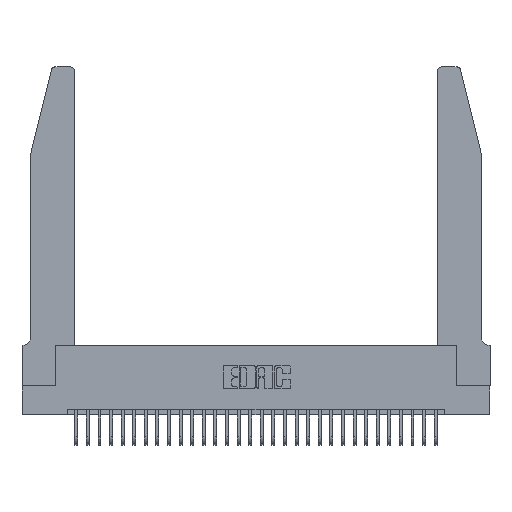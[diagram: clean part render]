
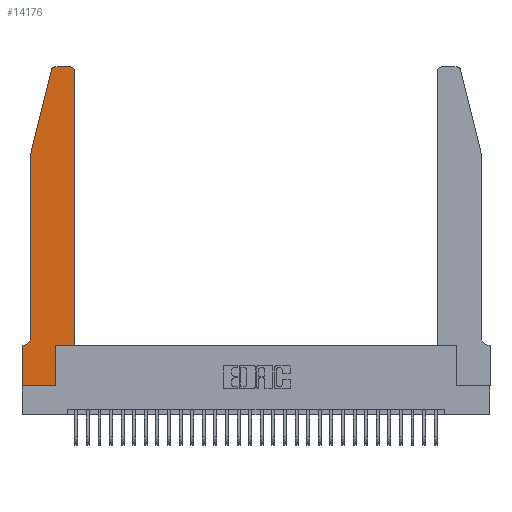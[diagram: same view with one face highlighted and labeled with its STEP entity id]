
A CAD part, top view. The second image highlights one B-rep face of the part: STEP entity #14176.
In plain terms, the highlighted planar face has unit normal (0, 0, 1).
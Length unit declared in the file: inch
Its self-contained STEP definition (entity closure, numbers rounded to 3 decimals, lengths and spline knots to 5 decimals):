
#219 = VERTEX_POINT ( 'NONE', #13088 ) ;
#711 = CARTESIAN_POINT ( 'NONE',  ( 0., 0.35, 0.37 ) ) ;
#771 = CARTESIAN_POINT ( 'NONE',  ( 0.284, 2.72, 0.37 ) ) ;
#917 = AXIS2_PLACEMENT_3D ( 'NONE', #13949, #31653, #6155 ) ;
#1237 = LINE ( 'NONE', #27225, #2818 ) ;
#1404 = EDGE_CURVE ( 'NONE', #24025, #219, #1237, .T. ) ;
#1499 = CARTESIAN_POINT ( 'NONE',  ( 0.0755, 2., 0.37 ) ) ;
#2459 = CARTESIAN_POINT ( 'NONE',  ( 0.25487, 2.72718, 0.37 ) ) ;
#2487 = ORIENTED_EDGE ( 'NONE', *, *, #15381, .T. ) ;
#2818 = VECTOR ( 'NONE', #19490, 39.37008 ) ;
#2945 = ORIENTED_EDGE ( 'NONE', *, *, #10457, .T. ) ;
#2950 = PLANE ( 'NONE',  #24536 ) ;
#3220 = DIRECTION ( 'NONE',  ( -1., 0., 0. ) ) ;
#3922 = EDGE_CURVE ( 'NONE', #29432, #16314, #8284, .T. ) ;
#4212 = DIRECTION ( 'NONE',  ( 0., -1., 0. ) ) ;
#4270 = ORIENTED_EDGE ( 'NONE', *, *, #27706, .T. ) ;
#4544 = CARTESIAN_POINT ( 'NONE',  ( 0., 0., 0.37 ) ) ;
#5168 = VERTEX_POINT ( 'NONE', #10893 ) ;
#5199 = EDGE_CURVE ( 'NONE', #18612, #29432, #10990, .T. ) ;
#5569 = LINE ( 'NONE', #15874, #29776 ) ;
#5787 = CIRCLE ( 'NONE', #917, 0.03 ) ;
#5905 = DIRECTION ( 'NONE',  ( 1., 0., 0. ) ) ;
#6045 = VERTEX_POINT ( 'NONE', #31660 ) ;
#6155 = DIRECTION ( 'NONE',  ( 1., 0., 0. ) ) ;
#7247 = AXIS2_PLACEMENT_3D ( 'NONE', #27006, #32751, #15137 ) ;
#7865 = CARTESIAN_POINT ( 'NONE',  ( 0.2865, 0., 0.37 ) ) ;
#8284 = CIRCLE ( 'NONE', #31487, 0.03 ) ;
#9076 = VERTEX_POINT ( 'NONE', #21941 ) ;
#9089 = EDGE_LOOP ( 'NONE', ( #11054, #27358, #19783, #16013, #18417, #4270, #27289, #14657, #15229, #17934, #2945, #2487 ) ) ;
#9290 = CARTESIAN_POINT ( 'NONE',  ( 0., 0., 0.37 ) ) ;
#9731 = VERTEX_POINT ( 'NONE', #18243 ) ;
#10457 = EDGE_CURVE ( 'NONE', #9731, #6045, #5569, .T. ) ;
#10893 = CARTESIAN_POINT ( 'NONE',  ( 0., 0.35, 0.37 ) ) ;
#10990 = LINE ( 'NONE', #31607, #28789 ) ;
#11047 = CARTESIAN_POINT ( 'NONE',  ( 0.0755, 2., 0.37 ) ) ;
#11054 = ORIENTED_EDGE ( 'NONE', *, *, #5199, .T. ) ;
#12285 = VERTEX_POINT ( 'NONE', #31798 ) ;
#12386 = VECTOR ( 'NONE', #4212, 39.37008 ) ;
#13088 = CARTESIAN_POINT ( 'NONE',  ( 0.2865, 0.35, 0.37 ) ) ;
#13202 = CARTESIAN_POINT ( 'NONE',  ( 0.4205, 2.75, 0.37 ) ) ;
#13949 = CARTESIAN_POINT ( 'NONE',  ( 0.4205, 2.72, 0.37 ) ) ;
#14176 = ADVANCED_FACE ( 'NONE', ( #15423 ), #2950, .T. ) ;
#14657 = ORIENTED_EDGE ( 'NONE', *, *, #22656, .T. ) ;
#14736 = CARTESIAN_POINT ( 'NONE',  ( 0., 0., 0.37 ) ) ;
#14869 = EDGE_CURVE ( 'NONE', #16314, #31996, #22487, .T. ) ;
#15137 = DIRECTION ( 'NONE',  ( -1., 0., 0. ) ) ;
#15229 = ORIENTED_EDGE ( 'NONE', *, *, #1404, .T. ) ;
#15381 = EDGE_CURVE ( 'NONE', #6045, #18612, #5787, .T. ) ;
#15392 = VECTOR ( 'NONE', #24279, 39.37008 ) ;
#15423 = FACE_OUTER_BOUND ( 'NONE', #9089, .T. ) ;
#15554 = LINE ( 'NONE', #4544, #12386 ) ;
#15874 = CARTESIAN_POINT ( 'NONE',  ( 0.4505, 0.35, 0.37 ) ) ;
#16013 = ORIENTED_EDGE ( 'NONE', *, *, #21296, .T. ) ;
#16299 = LINE ( 'NONE', #25764, #26205 ) ;
#16314 = VERTEX_POINT ( 'NONE', #2459 ) ;
#16662 = DIRECTION ( 'NONE',  ( -1., 0., 0. ) ) ;
#17136 = VECTOR ( 'NONE', #22157, 39.37008 ) ;
#17240 = LINE ( 'NONE', #14736, #20772 ) ;
#17299 = CIRCLE ( 'NONE', #7247, 0.07 ) ;
#17618 = DIRECTION ( 'NONE',  ( 1., 0., 0. ) ) ;
#17934 = ORIENTED_EDGE ( 'NONE', *, *, #26723, .T. ) ;
#18086 = DIRECTION ( 'NONE',  ( 0., 1., 0. ) ) ;
#18243 = CARTESIAN_POINT ( 'NONE',  ( 0.4505, 0.35, 0.37 ) ) ;
#18297 = CARTESIAN_POINT ( 'NONE',  ( 0.0755, 2., 0.37 ) ) ;
#18366 = DIRECTION ( 'NONE',  ( 0., -1., 0. ) ) ;
#18417 = ORIENTED_EDGE ( 'NONE', *, *, #21537, .T. ) ;
#18612 = VERTEX_POINT ( 'NONE', #13202 ) ;
#19490 = DIRECTION ( 'NONE',  ( 0., 1., 0. ) ) ;
#19659 = CARTESIAN_POINT ( 'NONE',  ( 0.4505, 0.35, 0.37 ) ) ;
#19783 = ORIENTED_EDGE ( 'NONE', *, *, #14869, .T. ) ;
#20772 = VECTOR ( 'NONE', #17618, 39.37008 ) ;
#20849 = DIRECTION ( 'NONE',  ( 1., 0., 0. ) ) ;
#21111 = DIRECTION ( 'NONE',  ( 0., 0., 1. ) ) ;
#21296 = EDGE_CURVE ( 'NONE', #31996, #9076, #27602, .T. ) ;
#21537 = EDGE_CURVE ( 'NONE', #9076, #12285, #17299, .T. ) ;
#21941 = CARTESIAN_POINT ( 'NONE',  ( 0.0755, 0.42, 0.37 ) ) ;
#22157 = DIRECTION ( 'NONE',  ( 1., 0., 0. ) ) ;
#22487 = LINE ( 'NONE', #1499, #15392 ) ;
#22656 = EDGE_CURVE ( 'NONE', #24385, #24025, #17240, .T. ) ;
#24025 = VERTEX_POINT ( 'NONE', #7865 ) ;
#24279 = DIRECTION ( 'NONE',  ( -0.239, -0.971, 0. ) ) ;
#24385 = VERTEX_POINT ( 'NONE', #9290 ) ;
#24536 = AXIS2_PLACEMENT_3D ( 'NONE', #711, #28444, #20849 ) ;
#24650 = LINE ( 'NONE', #19659, #17136 ) ;
#25635 = VECTOR ( 'NONE', #18366, 39.37008 ) ;
#25764 = CARTESIAN_POINT ( 'NONE',  ( 0.0755, 0.35, 0.37 ) ) ;
#26205 = VECTOR ( 'NONE', #3220, 39.37008 ) ;
#26628 = EDGE_CURVE ( 'NONE', #5168, #24385, #15554, .T. ) ;
#26723 = EDGE_CURVE ( 'NONE', #219, #9731, #24650, .T. ) ;
#27006 = CARTESIAN_POINT ( 'NONE',  ( 0.0055, 0.42, 0.37 ) ) ;
#27225 = CARTESIAN_POINT ( 'NONE',  ( 0.2865, 0.35, 0.37 ) ) ;
#27289 = ORIENTED_EDGE ( 'NONE', *, *, #26628, .T. ) ;
#27358 = ORIENTED_EDGE ( 'NONE', *, *, #3922, .T. ) ;
#27602 = LINE ( 'NONE', #11047, #25635 ) ;
#27706 = EDGE_CURVE ( 'NONE', #12285, #5168, #16299, .T. ) ;
#28444 = DIRECTION ( 'NONE',  ( 0., 0., 1. ) ) ;
#28789 = VECTOR ( 'NONE', #16662, 39.37008 ) ;
#29432 = VERTEX_POINT ( 'NONE', #29591 ) ;
#29591 = CARTESIAN_POINT ( 'NONE',  ( 0.284, 2.75, 0.37 ) ) ;
#29776 = VECTOR ( 'NONE', #18086, 39.37008 ) ;
#31487 = AXIS2_PLACEMENT_3D ( 'NONE', #771, #21111, #5905 ) ;
#31607 = CARTESIAN_POINT ( 'NONE',  ( 0.2605, 2.75, 0.37 ) ) ;
#31653 = DIRECTION ( 'NONE',  ( 0., 0., 1. ) ) ;
#31660 = CARTESIAN_POINT ( 'NONE',  ( 0.4505, 2.72, 0.37 ) ) ;
#31798 = CARTESIAN_POINT ( 'NONE',  ( 0.0055, 0.35, 0.37 ) ) ;
#31996 = VERTEX_POINT ( 'NONE', #18297 ) ;
#32751 = DIRECTION ( 'NONE',  ( 0., 0., -1. ) ) ;
